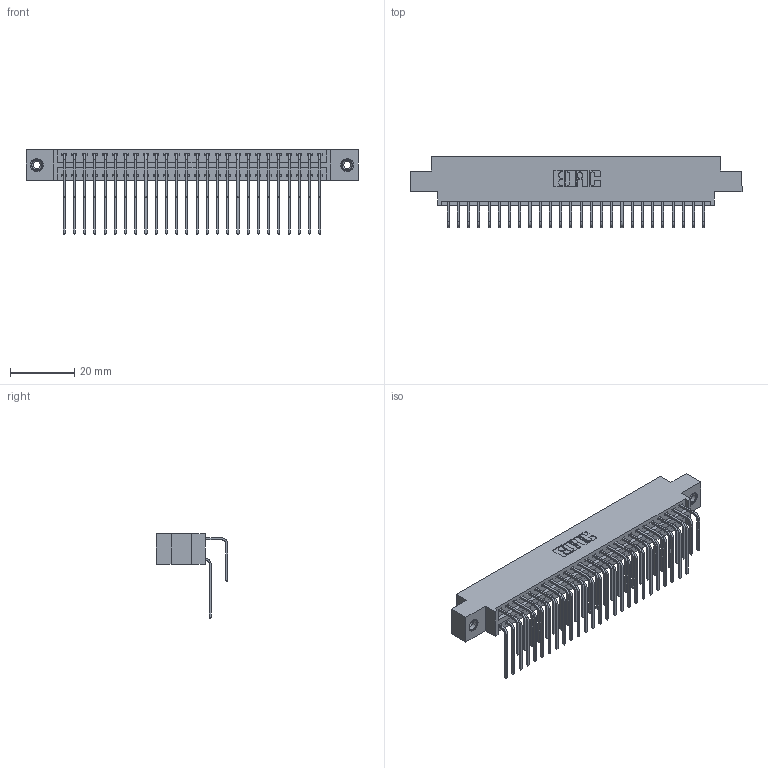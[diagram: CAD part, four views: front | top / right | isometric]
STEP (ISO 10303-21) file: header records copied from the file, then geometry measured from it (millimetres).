
FILE_DESCRIPTION (( 'STEP AP203' ), '1' );
FILE_NAME ('346-052-558-808.STEP', '2018-08-28T00:25:50', ( '' ), ( '' ), 'SwSTEP 2.0', 'SolidWorks 2016', '' );
FILE_SCHEMA (( 'CONFIG_CONTROL_DESIGN' ));
Length unit declared in the file: inch
Products named in the file (5): 346 Part_0.170 Offset - 0.156 Dia-TI; 345-292-001_558 559 Tail - 1; 345-292-001_558 Tail - 2; 345-250-001_345-250-003-102; 346-052-558-808
Assembly tree (55 placements, depth 2):
  346-052-558-808
    346 Part_0.170 Offset - 0.156 Dia-TI
    345-292-001_558 559 Tail - 1  x26
    345-292-001_558 Tail - 2  x26
    345-250-001_345-250-003-102  x2
Bounding box: 103.12 x 22.16 x 26.16 mm (x, y, z)
Volume: 10070.4 mm3; surface area: 15229.8 mm2
Topology: 55 solids, 55 shells, 2994 faces, 8849 edges, 5822 vertices
Faces by surface type: plane 2036, cylinder 942, cone 12, torus 4
Entity records: 22224 total; most frequent: CARTESIAN_POINT 3722, ORIENTED_EDGE 3598, DIRECTION 3329, EDGE_CURVE 1799, LINE 1503, VECTOR 1503, VERTEX_POINT 1192, AXIS2_PLACEMENT_3D 913
